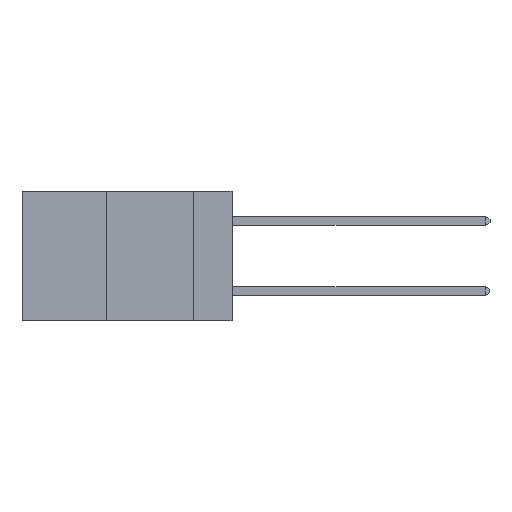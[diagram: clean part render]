
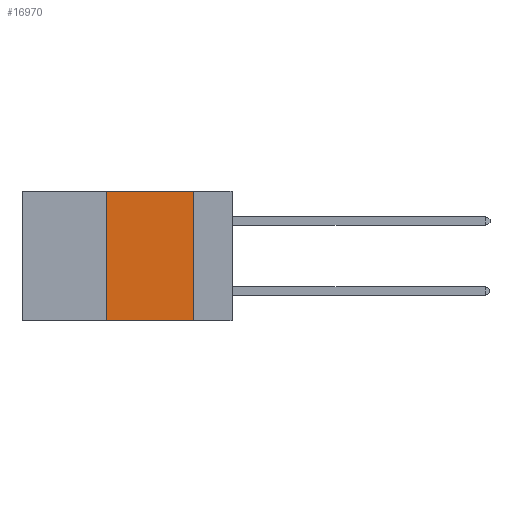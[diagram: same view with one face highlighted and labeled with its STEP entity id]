
A CAD part, left-side view. The second image highlights one B-rep face of the part: STEP entity #16970.
In plain terms, the highlighted planar face has unit normal (-1, 0, 0).
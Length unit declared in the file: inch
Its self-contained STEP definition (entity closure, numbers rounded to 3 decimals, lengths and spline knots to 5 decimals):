
#189 = ORIENTED_EDGE ( 'NONE', *, *, #16408, .T. ) ;
#1823 = LINE ( 'NONE', #6656, #9476 ) ;
#2406 = DIRECTION ( 'NONE',  ( 0., -1., 0. ) ) ;
#2652 = LINE ( 'NONE', #4455, #19543 ) ;
#3238 = ORIENTED_EDGE ( 'NONE', *, *, #19224, .F. ) ;
#3292 = CARTESIAN_POINT ( 'NONE',  ( 0., 0.36, -0.37 ) ) ;
#3406 = DIRECTION ( 'NONE',  ( 0., -1., 0. ) ) ;
#3792 = LINE ( 'NONE', #15427, #7628 ) ;
#4455 = CARTESIAN_POINT ( 'NONE',  ( 0., 0.11, 0. ) ) ;
#6508 = PLANE ( 'NONE',  #18733 ) ;
#6656 = CARTESIAN_POINT ( 'NONE',  ( 0., 0.36, 0. ) ) ;
#7107 = ORIENTED_EDGE ( 'NONE', *, *, #20832, .F. ) ;
#7543 = LINE ( 'NONE', #11588, #15221 ) ;
#7628 = VECTOR ( 'NONE', #2406, 39.37008 ) ;
#7820 = DIRECTION ( 'NONE',  ( 0., 0., -1. ) ) ;
#8116 = CARTESIAN_POINT ( 'NONE',  ( 0., 0.6, 0. ) ) ;
#8197 = CARTESIAN_POINT ( 'NONE',  ( 0., 0.11, 0. ) ) ;
#9476 = VECTOR ( 'NONE', #16409, 39.37008 ) ;
#9804 = FACE_OUTER_BOUND ( 'NONE', #16255, .T. ) ;
#11419 = DIRECTION ( 'NONE',  ( 0., 0., -1. ) ) ;
#11588 = CARTESIAN_POINT ( 'NONE',  ( 0., 0.6, -0.37 ) ) ;
#14733 = VERTEX_POINT ( 'NONE', #18300 ) ;
#15139 = VERTEX_POINT ( 'NONE', #20897 ) ;
#15221 = VECTOR ( 'NONE', #3406, 39.37008 ) ;
#15280 = VERTEX_POINT ( 'NONE', #3292 ) ;
#15427 = CARTESIAN_POINT ( 'NONE',  ( 0., 0.6, 0. ) ) ;
#16255 = EDGE_LOOP ( 'NONE', ( #19619, #7107, #3238, #189 ) ) ;
#16408 = EDGE_CURVE ( 'NONE', #15280, #15139, #7543, .T. ) ;
#16409 = DIRECTION ( 'NONE',  ( 0., 0., 1. ) ) ;
#16970 = ADVANCED_FACE ( 'NONE', ( #9804 ), #6508, .F. ) ;
#17509 = EDGE_CURVE ( 'NONE', #19185, #15139, #2652, .T. ) ;
#18300 = CARTESIAN_POINT ( 'NONE',  ( 0., 0.36, 0. ) ) ;
#18733 = AXIS2_PLACEMENT_3D ( 'NONE', #8116, #21204, #11419 ) ;
#19185 = VERTEX_POINT ( 'NONE', #8197 ) ;
#19224 = EDGE_CURVE ( 'NONE', #15280, #14733, #1823, .T. ) ;
#19543 = VECTOR ( 'NONE', #7820, 39.37008 ) ;
#19619 = ORIENTED_EDGE ( 'NONE', *, *, #17509, .F. ) ;
#20832 = EDGE_CURVE ( 'NONE', #14733, #19185, #3792, .T. ) ;
#20897 = CARTESIAN_POINT ( 'NONE',  ( 0., 0.11, -0.37 ) ) ;
#21204 = DIRECTION ( 'NONE',  ( 1., 0., 0. ) ) ;
